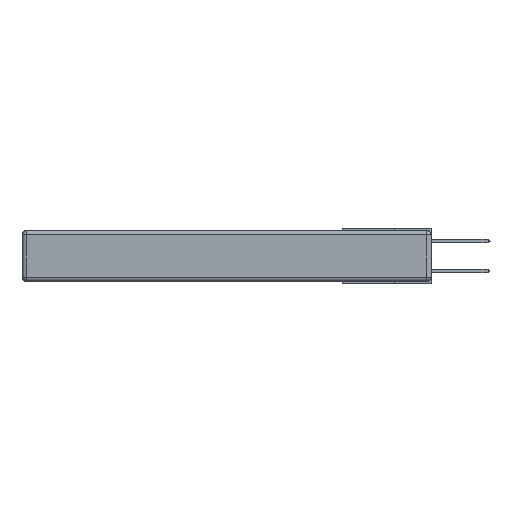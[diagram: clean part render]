
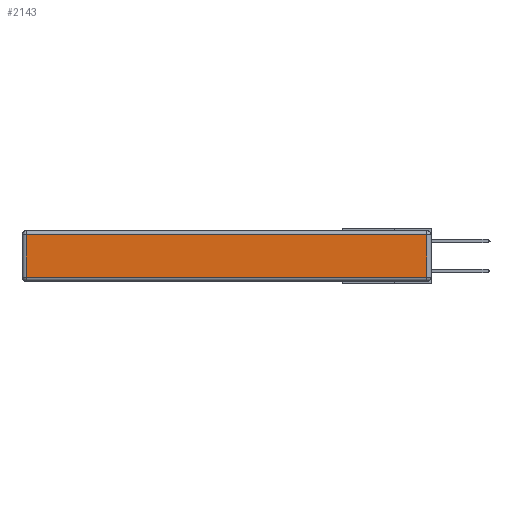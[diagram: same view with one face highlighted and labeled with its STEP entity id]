
A CAD part, left-side view. The second image highlights one B-rep face of the part: STEP entity #2143.
In plain terms, the highlighted planar face has unit normal (-1, 0, 0).
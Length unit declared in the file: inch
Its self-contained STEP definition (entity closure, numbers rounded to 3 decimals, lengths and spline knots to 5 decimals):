
#379 = VERTEX_POINT ( 'NONE', #8738 ) ;
#743 = DIRECTION ( 'NONE',  ( 0., 0., -1. ) ) ;
#1745 = DIRECTION ( 'NONE',  ( 0., 0., 1. ) ) ;
#1905 = DIRECTION ( 'NONE',  ( -1., 0., 0. ) ) ;
#2143 = ADVANCED_FACE ( 'NONE', ( #24348 ), #19840, .T. ) ;
#2263 = ORIENTED_EDGE ( 'NONE', *, *, #8794, .T. ) ;
#2745 = VERTEX_POINT ( 'NONE', #7560 ) ;
#3526 = VECTOR ( 'NONE', #7827, 39.37008 ) ;
#3742 = CARTESIAN_POINT ( 'NONE',  ( 0., 0.03, -0.313 ) ) ;
#4475 = VERTEX_POINT ( 'NONE', #3742 ) ;
#6977 = DIRECTION ( 'NONE',  ( 0., -1., 0. ) ) ;
#7098 = LINE ( 'NONE', #7626, #3526 ) ;
#7560 = CARTESIAN_POINT ( 'NONE',  ( 0., 0.03, -0.03 ) ) ;
#7627 = VERTEX_POINT ( 'NONE', #24175 ) ;
#7626 = CARTESIAN_POINT ( 'NONE',  ( 0., 2.75, -0.03 ) ) ;
#7827 = DIRECTION ( 'NONE',  ( 0., 1., 0. ) ) ;
#7920 = ORIENTED_EDGE ( 'NONE', *, *, #18235, .T. ) ;
#8738 = CARTESIAN_POINT ( 'NONE',  ( 0., 2.72, -0.03 ) ) ;
#8764 = VECTOR ( 'NONE', #743, 39.37008 ) ;
#8794 = EDGE_CURVE ( 'NONE', #379, #7627, #27692, .T. ) ;
#9416 = LINE ( 'NONE', #24932, #20445 ) ;
#10681 = EDGE_LOOP ( 'NONE', ( #7920, #14184, #29145, #2263 ) ) ;
#11447 = CARTESIAN_POINT ( 'NONE',  ( 0., 0., -0.313 ) ) ;
#13335 = EDGE_CURVE ( 'NONE', #4475, #2745, #9416, .T. ) ;
#14184 = ORIENTED_EDGE ( 'NONE', *, *, #13335, .T. ) ;
#14601 = VECTOR ( 'NONE', #6977, 39.37008 ) ;
#17377 = CARTESIAN_POINT ( 'NONE',  ( 0., 2.72, -0.343 ) ) ;
#17449 = LINE ( 'NONE', #11447, #14601 ) ;
#18235 = EDGE_CURVE ( 'NONE', #7627, #4475, #17449, .T. ) ;
#19840 = PLANE ( 'NONE',  #25178 ) ;
#20445 = VECTOR ( 'NONE', #1745, 39.37008 ) ;
#22109 = DIRECTION ( 'NONE',  ( 0., 0., 1. ) ) ;
#23357 = EDGE_CURVE ( 'NONE', #2745, #379, #7098, .T. ) ;
#24175 = CARTESIAN_POINT ( 'NONE',  ( 0., 2.72, -0.313 ) ) ;
#24348 = FACE_OUTER_BOUND ( 'NONE', #10681, .T. ) ;
#24625 = CARTESIAN_POINT ( 'NONE',  ( 0., 0., -0.343 ) ) ;
#24932 = CARTESIAN_POINT ( 'NONE',  ( 0., 0.03, -0.343 ) ) ;
#25178 = AXIS2_PLACEMENT_3D ( 'NONE', #24625, #1905, #22109 ) ;
#27692 = LINE ( 'NONE', #17377, #8764 ) ;
#29145 = ORIENTED_EDGE ( 'NONE', *, *, #23357, .T. ) ;
